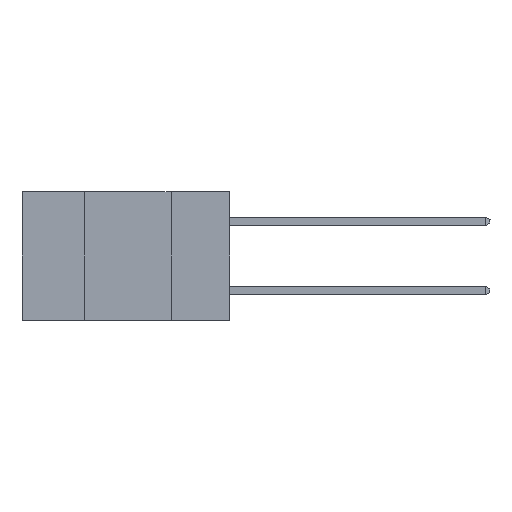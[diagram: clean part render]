
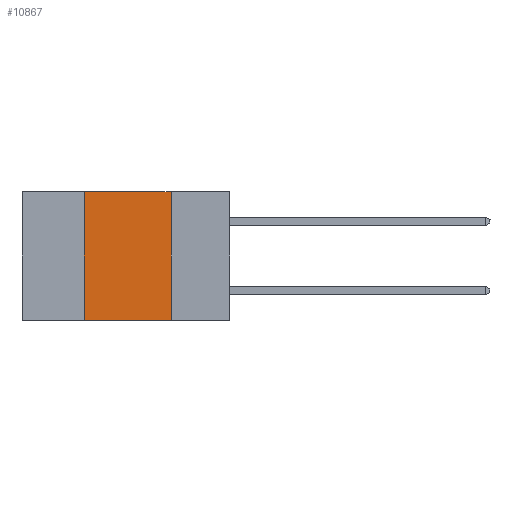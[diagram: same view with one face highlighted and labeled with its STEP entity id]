
A CAD part, left-side view. The second image highlights one B-rep face of the part: STEP entity #10867.
In plain terms, the highlighted planar face has unit normal (-1, 0, 0).
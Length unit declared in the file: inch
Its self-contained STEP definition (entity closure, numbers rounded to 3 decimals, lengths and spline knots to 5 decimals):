
#88 = VECTOR ( 'NONE', #1281, 39.37008 ) ;
#182 = EDGE_CURVE ( 'NONE', #15421, #6985, #6462, .T. ) ;
#1281 = DIRECTION ( 'NONE',  ( 0., -1., 0. ) ) ;
#1865 = CARTESIAN_POINT ( 'NONE',  ( 0., 0.17, -0.37 ) ) ;
#2394 = DIRECTION ( 'NONE',  ( 0., -1., 0. ) ) ;
#2737 = FACE_OUTER_BOUND ( 'NONE', #13405, .T. ) ;
#2818 = CARTESIAN_POINT ( 'NONE',  ( 0., 0.6, 0. ) ) ;
#3510 = LINE ( 'NONE', #3970, #17417 ) ;
#3970 = CARTESIAN_POINT ( 'NONE',  ( 0., 0.17, 0. ) ) ;
#4438 = EDGE_CURVE ( 'NONE', #15421, #17476, #8917, .T. ) ;
#5475 = CARTESIAN_POINT ( 'NONE',  ( 0., 0.17, 0. ) ) ;
#5492 = ORIENTED_EDGE ( 'NONE', *, *, #17708, .F. ) ;
#5721 = VECTOR ( 'NONE', #9346, 39.37008 ) ;
#5862 = LINE ( 'NONE', #2818, #88 ) ;
#6421 = EDGE_CURVE ( 'NONE', #6985, #18657, #5862, .T. ) ;
#6462 = LINE ( 'NONE', #13860, #5721 ) ;
#6985 = VERTEX_POINT ( 'NONE', #14793 ) ;
#7771 = CARTESIAN_POINT ( 'NONE',  ( 0., 0.6, -0.37 ) ) ;
#8917 = LINE ( 'NONE', #7771, #14911 ) ;
#9346 = DIRECTION ( 'NONE',  ( 0., 0., 1. ) ) ;
#9382 = CARTESIAN_POINT ( 'NONE',  ( 0., 0.6, 0. ) ) ;
#9772 = ORIENTED_EDGE ( 'NONE', *, *, #4438, .T. ) ;
#10867 = ADVANCED_FACE ( 'NONE', ( #2737 ), #16722, .F. ) ;
#11215 = CARTESIAN_POINT ( 'NONE',  ( 0., 0.42, -0.37 ) ) ;
#11677 = ORIENTED_EDGE ( 'NONE', *, *, #182, .F. ) ;
#13405 = EDGE_LOOP ( 'NONE', ( #5492, #18464, #11677, #9772 ) ) ;
#13703 = DIRECTION ( 'NONE',  ( 1., 0., 0. ) ) ;
#13836 = DIRECTION ( 'NONE',  ( 0., 0., -1. ) ) ;
#13860 = CARTESIAN_POINT ( 'NONE',  ( 0., 0.42, 0. ) ) ;
#14793 = CARTESIAN_POINT ( 'NONE',  ( 0., 0.42, 0. ) ) ;
#14911 = VECTOR ( 'NONE', #2394, 39.37008 ) ;
#15421 = VERTEX_POINT ( 'NONE', #11215 ) ;
#16722 = PLANE ( 'NONE',  #18345 ) ;
#17417 = VECTOR ( 'NONE', #17533, 39.37008 ) ;
#17476 = VERTEX_POINT ( 'NONE', #1865 ) ;
#17533 = DIRECTION ( 'NONE',  ( 0., 0., -1. ) ) ;
#17708 = EDGE_CURVE ( 'NONE', #18657, #17476, #3510, .T. ) ;
#18345 = AXIS2_PLACEMENT_3D ( 'NONE', #9382, #13703, #13836 ) ;
#18464 = ORIENTED_EDGE ( 'NONE', *, *, #6421, .F. ) ;
#18657 = VERTEX_POINT ( 'NONE', #5475 ) ;
